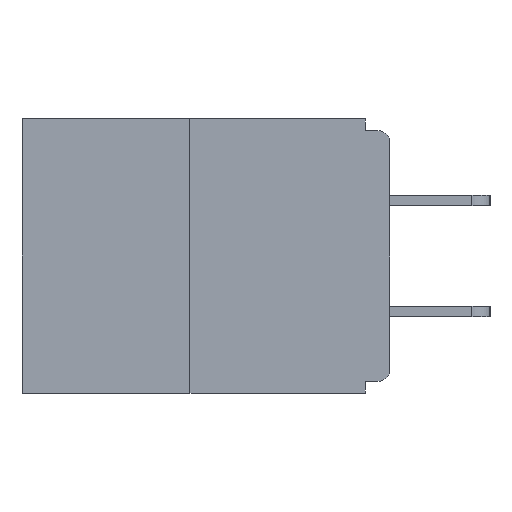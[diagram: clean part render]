
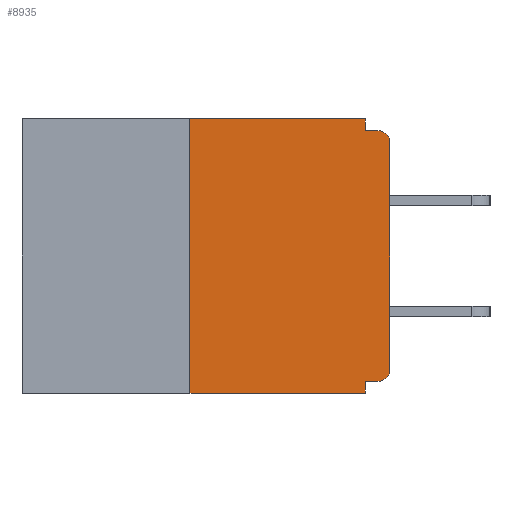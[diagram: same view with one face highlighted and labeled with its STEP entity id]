
A CAD part, left-side view. The second image highlights one B-rep face of the part: STEP entity #8935.
In plain terms, the highlighted planar face has unit normal (-1, 0, 0).
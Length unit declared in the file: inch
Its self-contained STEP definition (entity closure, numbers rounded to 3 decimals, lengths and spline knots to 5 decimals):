
#84 = CARTESIAN_POINT ( 'NONE',  ( 0., 0.25, -0.343 ) ) ;
#800 = ORIENTED_EDGE ( 'NONE', *, *, #20272, .T. ) ;
#878 = EDGE_CURVE ( 'NONE', #22646, #16929, #23613, .T. ) ;
#1017 = VECTOR ( 'NONE', #10802, 39.37008 ) ;
#1148 = VERTEX_POINT ( 'NONE', #17990 ) ;
#1183 = CARTESIAN_POINT ( 'NONE',  ( 0., 0.015, -0.328 ) ) ;
#2328 = CARTESIAN_POINT ( 'NONE',  ( 0., 0.015, -0.015 ) ) ;
#2689 = ORIENTED_EDGE ( 'NONE', *, *, #7444, .F. ) ;
#3483 = DIRECTION ( 'NONE',  ( -1., 0., 0. ) ) ;
#4167 = ORIENTED_EDGE ( 'NONE', *, *, #5173, .F. ) ;
#4408 = CARTESIAN_POINT ( 'NONE',  ( 0., 0., -0.015 ) ) ;
#5063 = EDGE_CURVE ( 'NONE', #23088, #25000, #9807, .T. ) ;
#5173 = EDGE_CURVE ( 'NONE', #5393, #25071, #8853, .T. ) ;
#5393 = VERTEX_POINT ( 'NONE', #15238 ) ;
#6038 = LINE ( 'NONE', #16010, #12202 ) ;
#6450 = LINE ( 'NONE', #10578, #8633 ) ;
#6856 = ORIENTED_EDGE ( 'NONE', *, *, #9975, .T. ) ;
#7226 = DIRECTION ( 'NONE',  ( 0., 0., -1. ) ) ;
#7322 = VECTOR ( 'NONE', #7226, 39.37008 ) ;
#7444 = EDGE_CURVE ( 'NONE', #16980, #23088, #11857, .T. ) ;
#7478 = CARTESIAN_POINT ( 'NONE',  ( 0., 0.015, -0.03 ) ) ;
#8427 = DIRECTION ( 'NONE',  ( -1., 0., 0. ) ) ;
#8633 = VECTOR ( 'NONE', #16273, 39.37008 ) ;
#8753 = VECTOR ( 'NONE', #18449, 39.37008 ) ;
#8853 = LINE ( 'NONE', #4408, #11012 ) ;
#8935 = ADVANCED_FACE ( 'NONE', ( #11126 ), #17179, .F. ) ;
#9190 = DIRECTION ( 'NONE',  ( 0., 0., -1. ) ) ;
#9776 = CARTESIAN_POINT ( 'NONE',  ( 0., 0., -0.03 ) ) ;
#9807 = LINE ( 'NONE', #19058, #7322 ) ;
#9975 = EDGE_CURVE ( 'NONE', #16980, #1148, #18797, .T. ) ;
#9993 = EDGE_LOOP ( 'NONE', ( #12938, #13132, #800, #14480, #2689, #6856, #20251, #18742, #4167, #18234 ) ) ;
#10358 = DIRECTION ( 'NONE',  ( 0., -1., 0. ) ) ;
#10578 = CARTESIAN_POINT ( 'NONE',  ( 0., 0.031, 0. ) ) ;
#10595 = CARTESIAN_POINT ( 'NONE',  ( 0., 0., 0. ) ) ;
#10802 = DIRECTION ( 'NONE',  ( 0., -1., 0. ) ) ;
#11012 = VECTOR ( 'NONE', #10358, 39.37008 ) ;
#11126 = FACE_OUTER_BOUND ( 'NONE', #9993, .T. ) ;
#11329 = DIRECTION ( 'NONE',  ( 0., 0., -1. ) ) ;
#11857 = LINE ( 'NONE', #15076, #21443 ) ;
#12202 = VECTOR ( 'NONE', #14109, 39.37008 ) ;
#12462 = AXIS2_PLACEMENT_3D ( 'NONE', #21161, #23181, #11329 ) ;
#12486 = AXIS2_PLACEMENT_3D ( 'NONE', #7478, #3483, #9190 ) ;
#12625 = EDGE_CURVE ( 'NONE', #1148, #13657, #19072, .T. ) ;
#12938 = ORIENTED_EDGE ( 'NONE', *, *, #24411, .F. ) ;
#13132 = ORIENTED_EDGE ( 'NONE', *, *, #878, .F. ) ;
#13657 = VERTEX_POINT ( 'NONE', #9776 ) ;
#14109 = DIRECTION ( 'NONE',  ( 0., -1., 0. ) ) ;
#14480 = ORIENTED_EDGE ( 'NONE', *, *, #5063, .F. ) ;
#14989 = DIRECTION ( 'NONE',  ( 0., 1., 0. ) ) ;
#15076 = CARTESIAN_POINT ( 'NONE',  ( 0., 0., -0.328 ) ) ;
#15238 = CARTESIAN_POINT ( 'NONE',  ( 0., 0.031, -0.015 ) ) ;
#15717 = CARTESIAN_POINT ( 'NONE',  ( 0., 0.031, -0.343 ) ) ;
#15943 = EDGE_CURVE ( 'NONE', #13657, #25071, #19876, .T. ) ;
#16010 = CARTESIAN_POINT ( 'NONE',  ( 0., 0.46, 0. ) ) ;
#16273 = DIRECTION ( 'NONE',  ( 0., 0., -1. ) ) ;
#16363 = DIRECTION ( 'NONE',  ( 0., 0., -1. ) ) ;
#16929 = VERTEX_POINT ( 'NONE', #20357 ) ;
#16980 = VERTEX_POINT ( 'NONE', #1183 ) ;
#17179 = PLANE ( 'NONE',  #12462 ) ;
#17990 = CARTESIAN_POINT ( 'NONE',  ( 0., 0., -0.313 ) ) ;
#18202 = VERTEX_POINT ( 'NONE', #24102 ) ;
#18234 = ORIENTED_EDGE ( 'NONE', *, *, #22825, .F. ) ;
#18449 = DIRECTION ( 'NONE',  ( 0., 0., 1. ) ) ;
#18742 = ORIENTED_EDGE ( 'NONE', *, *, #15943, .T. ) ;
#18797 = CIRCLE ( 'NONE', #18937, 0.015 ) ;
#18937 = AXIS2_PLACEMENT_3D ( 'NONE', #20265, #8427, #16363 ) ;
#19058 = CARTESIAN_POINT ( 'NONE',  ( 0., 0.031, -0.343 ) ) ;
#19072 = LINE ( 'NONE', #10595, #19715 ) ;
#19715 = VECTOR ( 'NONE', #24444, 39.37008 ) ;
#19876 = CIRCLE ( 'NONE', #12486, 0.015 ) ;
#20251 = ORIENTED_EDGE ( 'NONE', *, *, #12625, .T. ) ;
#20265 = CARTESIAN_POINT ( 'NONE',  ( 0., 0.015, -0.313 ) ) ;
#20272 = EDGE_CURVE ( 'NONE', #22646, #25000, #22042, .T. ) ;
#20357 = CARTESIAN_POINT ( 'NONE',  ( 0., 0.25, 0. ) ) ;
#21099 = CARTESIAN_POINT ( 'NONE',  ( 0., 0.031, -0.328 ) ) ;
#21161 = CARTESIAN_POINT ( 'NONE',  ( 0., 0.46, 0. ) ) ;
#21443 = VECTOR ( 'NONE', #14989, 39.37008 ) ;
#22042 = LINE ( 'NONE', #22636, #1017 ) ;
#22636 = CARTESIAN_POINT ( 'NONE',  ( 0., 0.46, -0.343 ) ) ;
#22646 = VERTEX_POINT ( 'NONE', #84 ) ;
#22825 = EDGE_CURVE ( 'NONE', #18202, #5393, #6450, .T. ) ;
#23088 = VERTEX_POINT ( 'NONE', #21099 ) ;
#23181 = DIRECTION ( 'NONE',  ( 1., 0., 0. ) ) ;
#23613 = LINE ( 'NONE', #24258, #8753 ) ;
#24102 = CARTESIAN_POINT ( 'NONE',  ( 0., 0.031, 0. ) ) ;
#24258 = CARTESIAN_POINT ( 'NONE',  ( 0., 0.25, 0. ) ) ;
#24411 = EDGE_CURVE ( 'NONE', #16929, #18202, #6038, .T. ) ;
#24444 = DIRECTION ( 'NONE',  ( 0., 0., 1. ) ) ;
#25000 = VERTEX_POINT ( 'NONE', #15717 ) ;
#25071 = VERTEX_POINT ( 'NONE', #2328 ) ;
